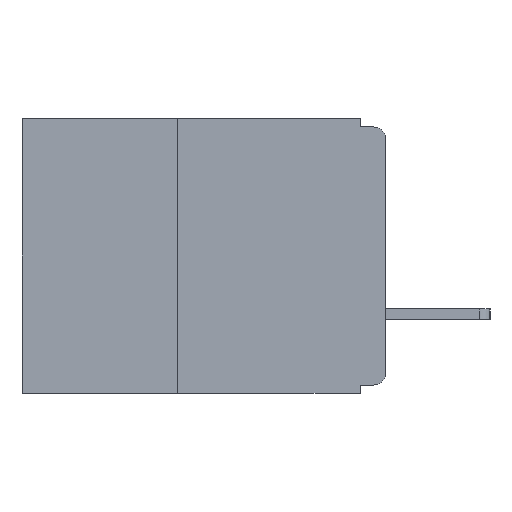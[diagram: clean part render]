
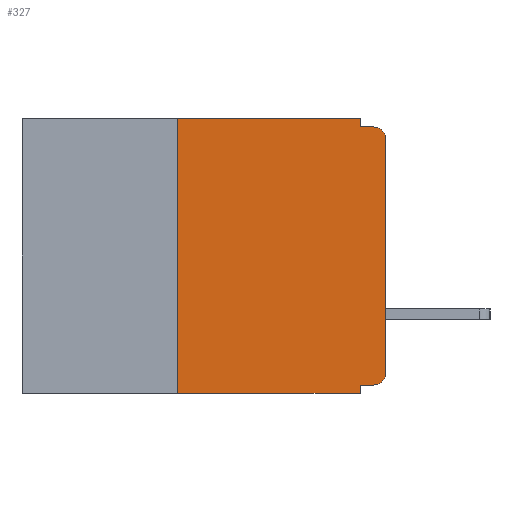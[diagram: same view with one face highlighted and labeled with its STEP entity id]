
A CAD part, left-side view. The second image highlights one B-rep face of the part: STEP entity #327.
In plain terms, the highlighted planar face has unit normal (-1, 0, 0).
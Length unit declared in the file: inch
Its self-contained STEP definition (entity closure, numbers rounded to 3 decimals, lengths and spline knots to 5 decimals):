
#327 = ADVANCED_FACE ( 'NONE', ( #17204 ), #15880, .F. ) ;
#840 = VERTEX_POINT ( 'NONE', #10866 ) ;
#850 = VECTOR ( 'NONE', #12688, 39.37008 ) ;
#899 = DIRECTION ( 'NONE',  ( 1., 0., 0. ) ) ;
#1216 = DIRECTION ( 'NONE',  ( -1., 0., 0. ) ) ;
#1285 = CARTESIAN_POINT ( 'NONE',  ( 0., 0.25, -0.33 ) ) ;
#1442 = AXIS2_PLACEMENT_3D ( 'NONE', #2448, #14003, #4089 ) ;
#1738 = ORIENTED_EDGE ( 'NONE', *, *, #13082, .T. ) ;
#1753 = VERTEX_POINT ( 'NONE', #20828 ) ;
#2253 = EDGE_CURVE ( 'NONE', #9783, #3324, #17929, .T. ) ;
#2278 = EDGE_CURVE ( 'NONE', #1753, #13190, #12474, .T. ) ;
#2448 = CARTESIAN_POINT ( 'NONE',  ( 0., 0.015, -0.025 ) ) ;
#2751 = CARTESIAN_POINT ( 'NONE',  ( 0., 0., -0.305 ) ) ;
#3036 = CARTESIAN_POINT ( 'NONE',  ( 0., 0.031, -0.33 ) ) ;
#3188 = VECTOR ( 'NONE', #7470, 39.37008 ) ;
#3220 = LINE ( 'NONE', #19002, #19789 ) ;
#3324 = VERTEX_POINT ( 'NONE', #21120 ) ;
#3808 = EDGE_CURVE ( 'NONE', #13190, #15244, #7200, .T. ) ;
#3868 = VECTOR ( 'NONE', #10495, 39.37008 ) ;
#4069 = CARTESIAN_POINT ( 'NONE',  ( 0., 0.031, -0.32 ) ) ;
#4089 = DIRECTION ( 'NONE',  ( 0., 0., -1. ) ) ;
#5043 = VECTOR ( 'NONE', #12885, 39.37008 ) ;
#5225 = ORIENTED_EDGE ( 'NONE', *, *, #15802, .F. ) ;
#5865 = EDGE_CURVE ( 'NONE', #6439, #9783, #15255, .T. ) ;
#6232 = CARTESIAN_POINT ( 'NONE',  ( 0., 0., -0.32 ) ) ;
#6326 = VERTEX_POINT ( 'NONE', #20606 ) ;
#6421 = VERTEX_POINT ( 'NONE', #12576 ) ;
#6439 = VERTEX_POINT ( 'NONE', #12718 ) ;
#6572 = EDGE_CURVE ( 'NONE', #20777, #6421, #6682, .T. ) ;
#6682 = LINE ( 'NONE', #3036, #19383 ) ;
#7200 = LINE ( 'NONE', #10791, #20407 ) ;
#7300 = CARTESIAN_POINT ( 'NONE',  ( 0., 0., -0.01 ) ) ;
#7470 = DIRECTION ( 'NONE',  ( 0., 0., -1. ) ) ;
#7906 = DIRECTION ( 'NONE',  ( 0., 0., 1. ) ) ;
#8285 = LINE ( 'NONE', #7300, #3868 ) ;
#9783 = VERTEX_POINT ( 'NONE', #13655 ) ;
#9894 = ORIENTED_EDGE ( 'NONE', *, *, #21281, .F. ) ;
#10014 = ORIENTED_EDGE ( 'NONE', *, *, #2253, .F. ) ;
#10114 = AXIS2_PLACEMENT_3D ( 'NONE', #19839, #1216, #20982 ) ;
#10495 = DIRECTION ( 'NONE',  ( 0., -1., 0. ) ) ;
#10755 = DIRECTION ( 'NONE',  ( 0., -1., 0. ) ) ;
#10776 = AXIS2_PLACEMENT_3D ( 'NONE', #15906, #899, #21405 ) ;
#10791 = CARTESIAN_POINT ( 'NONE',  ( 0., 0., 0. ) ) ;
#10856 = VECTOR ( 'NONE', #7906, 39.37008 ) ;
#10866 = CARTESIAN_POINT ( 'NONE',  ( 0., 0.015, -0.01 ) ) ;
#12202 = ORIENTED_EDGE ( 'NONE', *, *, #5865, .F. ) ;
#12474 = CIRCLE ( 'NONE', #10114, 0.015 ) ;
#12576 = CARTESIAN_POINT ( 'NONE',  ( 0., 0.031, -0.33 ) ) ;
#12688 = DIRECTION ( 'NONE',  ( 0., -1., 0. ) ) ;
#12704 = ORIENTED_EDGE ( 'NONE', *, *, #6572, .F. ) ;
#12718 = CARTESIAN_POINT ( 'NONE',  ( 0., 0.25, -0.33 ) ) ;
#12729 = EDGE_CURVE ( 'NONE', #1753, #20777, #18247, .T. ) ;
#12885 = DIRECTION ( 'NONE',  ( 0., 1., 0. ) ) ;
#13082 = EDGE_CURVE ( 'NONE', #6439, #6421, #3220, .T. ) ;
#13190 = VERTEX_POINT ( 'NONE', #2751 ) ;
#13285 = ORIENTED_EDGE ( 'NONE', *, *, #16392, .T. ) ;
#13655 = CARTESIAN_POINT ( 'NONE',  ( 0., 0.25, 0. ) ) ;
#14003 = DIRECTION ( 'NONE',  ( -1., 0., 0. ) ) ;
#14486 = ORIENTED_EDGE ( 'NONE', *, *, #3808, .T. ) ;
#15158 = ORIENTED_EDGE ( 'NONE', *, *, #12729, .F. ) ;
#15244 = VERTEX_POINT ( 'NONE', #19724 ) ;
#15255 = LINE ( 'NONE', #1285, #10856 ) ;
#15802 = EDGE_CURVE ( 'NONE', #6326, #840, #8285, .T. ) ;
#15871 = LINE ( 'NONE', #17397, #3188 ) ;
#15880 = PLANE ( 'NONE',  #10776 ) ;
#15906 = CARTESIAN_POINT ( 'NONE',  ( 0., 0.437, 0. ) ) ;
#16392 = EDGE_CURVE ( 'NONE', #15244, #840, #18344, .T. ) ;
#17090 = EDGE_LOOP ( 'NONE', ( #14486, #13285, #5225, #9894, #10014, #12202, #1738, #12704, #15158, #20634 ) ) ;
#17204 = FACE_OUTER_BOUND ( 'NONE', #17090, .T. ) ;
#17397 = CARTESIAN_POINT ( 'NONE',  ( 0., 0.031, 0. ) ) ;
#17502 = CARTESIAN_POINT ( 'NONE',  ( 0., 0.437, 0. ) ) ;
#17929 = LINE ( 'NONE', #17502, #850 ) ;
#18247 = LINE ( 'NONE', #6232, #5043 ) ;
#18344 = CIRCLE ( 'NONE', #1442, 0.015 ) ;
#19002 = CARTESIAN_POINT ( 'NONE',  ( 0., 0.437, -0.33 ) ) ;
#19383 = VECTOR ( 'NONE', #21283, 39.37008 ) ;
#19724 = CARTESIAN_POINT ( 'NONE',  ( 0., 0., -0.025 ) ) ;
#19789 = VECTOR ( 'NONE', #10755, 39.37008 ) ;
#19839 = CARTESIAN_POINT ( 'NONE',  ( 0., 0.015, -0.305 ) ) ;
#20407 = VECTOR ( 'NONE', #20708, 39.37008 ) ;
#20606 = CARTESIAN_POINT ( 'NONE',  ( 0., 0.031, -0.01 ) ) ;
#20634 = ORIENTED_EDGE ( 'NONE', *, *, #2278, .T. ) ;
#20708 = DIRECTION ( 'NONE',  ( 0., 0., 1. ) ) ;
#20777 = VERTEX_POINT ( 'NONE', #4069 ) ;
#20828 = CARTESIAN_POINT ( 'NONE',  ( 0., 0.015, -0.32 ) ) ;
#20982 = DIRECTION ( 'NONE',  ( 0., 0., -1. ) ) ;
#21120 = CARTESIAN_POINT ( 'NONE',  ( 0., 0.031, 0. ) ) ;
#21281 = EDGE_CURVE ( 'NONE', #3324, #6326, #15871, .T. ) ;
#21283 = DIRECTION ( 'NONE',  ( 0., 0., -1. ) ) ;
#21405 = DIRECTION ( 'NONE',  ( 0., 0., -1. ) ) ;
